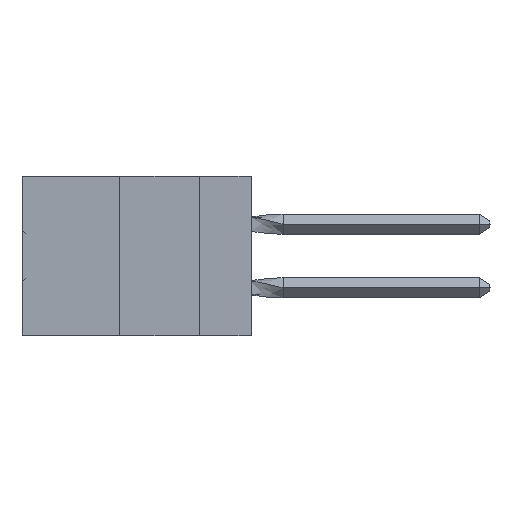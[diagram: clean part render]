
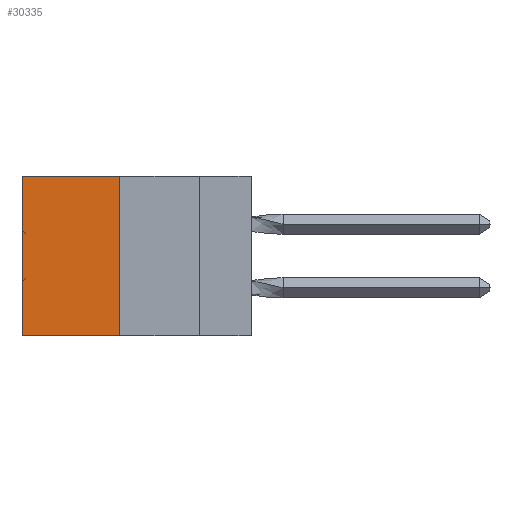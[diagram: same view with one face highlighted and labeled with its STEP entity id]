
A CAD part, left-side view. The second image highlights one B-rep face of the part: STEP entity #30335.
In plain terms, the highlighted planar face has unit normal (-1, 0, 0).
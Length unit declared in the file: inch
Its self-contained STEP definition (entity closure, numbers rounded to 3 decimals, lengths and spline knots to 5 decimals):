
#243 = EDGE_CURVE ( 'NONE', #32287, #43782, #18036, .T. ) ;
#2959 = ORIENTED_EDGE ( 'NONE', *, *, #51736, .F. ) ;
#6309 = VECTOR ( 'NONE', #26274, 39.37008 ) ;
#6877 = EDGE_CURVE ( 'NONE', #47929, #43782, #52965, .T. ) ;
#7078 = DIRECTION ( 'NONE',  ( 0., 0., -1. ) ) ;
#7112 = AXIS2_PLACEMENT_3D ( 'NONE', #16033, #40671, #7078 ) ;
#7266 = VERTEX_POINT ( 'NONE', #16038 ) ;
#7439 = PLANE ( 'NONE',  #7112 ) ;
#8695 = DIRECTION ( 'NONE',  ( 0., 1., 0. ) ) ;
#15142 = FACE_OUTER_BOUND ( 'NONE', #43622, .T. ) ;
#15678 = ORIENTED_EDGE ( 'NONE', *, *, #6877, .T. ) ;
#16033 = CARTESIAN_POINT ( 'NONE',  ( 0.305, 0.413, -0.5 ) ) ;
#16038 = CARTESIAN_POINT ( 'NONE',  ( 0.305, 0.413, 0. ) ) ;
#18036 = LINE ( 'NONE', #45262, #50277 ) ;
#20124 = DIRECTION ( 'NONE',  ( 0., 1., 0. ) ) ;
#21845 = CARTESIAN_POINT ( 'NONE',  ( 0.305, 0.413, -0.5 ) ) ;
#22319 = LINE ( 'NONE', #50946, #40040 ) ;
#25122 = CARTESIAN_POINT ( 'NONE',  ( 0.305, 0.72, -0.5 ) ) ;
#26274 = DIRECTION ( 'NONE',  ( 0., 0., -1. ) ) ;
#29343 = ORIENTED_EDGE ( 'NONE', *, *, #30774, .T. ) ;
#30335 = ADVANCED_FACE ( 'NONE', ( #15142 ), #7439, .F. ) ;
#30774 = EDGE_CURVE ( 'NONE', #7266, #47929, #22319, .T. ) ;
#32287 = VERTEX_POINT ( 'NONE', #44405 ) ;
#33994 = LINE ( 'NONE', #21845, #6309 ) ;
#35037 = CARTESIAN_POINT ( 'NONE',  ( 0.305, 0.72, 0. ) ) ;
#37731 = DIRECTION ( 'NONE',  ( 0., 0., -1. ) ) ;
#40040 = VECTOR ( 'NONE', #8695, 39.37008 ) ;
#40671 = DIRECTION ( 'NONE',  ( 1., 0., 0. ) ) ;
#41457 = ORIENTED_EDGE ( 'NONE', *, *, #243, .F. ) ;
#43622 = EDGE_LOOP ( 'NONE', ( #15678, #41457, #2959, #29343 ) ) ;
#43742 = VECTOR ( 'NONE', #37731, 39.37008 ) ;
#43782 = VERTEX_POINT ( 'NONE', #51047 ) ;
#44405 = CARTESIAN_POINT ( 'NONE',  ( 0.305, 0.413, -0.5 ) ) ;
#45262 = CARTESIAN_POINT ( 'NONE',  ( 0.305, 0.413, -0.5 ) ) ;
#47929 = VERTEX_POINT ( 'NONE', #35037 ) ;
#50277 = VECTOR ( 'NONE', #20124, 39.37008 ) ;
#50946 = CARTESIAN_POINT ( 'NONE',  ( 0.305, 0.413, 0. ) ) ;
#51047 = CARTESIAN_POINT ( 'NONE',  ( 0.305, 0.72, -0.5 ) ) ;
#51736 = EDGE_CURVE ( 'NONE', #7266, #32287, #33994, .T. ) ;
#52965 = LINE ( 'NONE', #25122, #43742 ) ;
